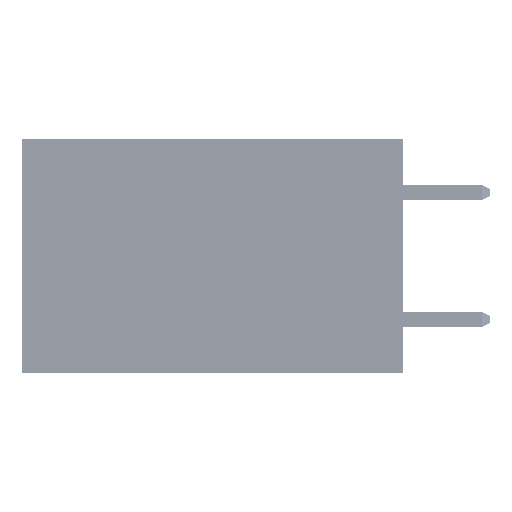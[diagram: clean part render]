
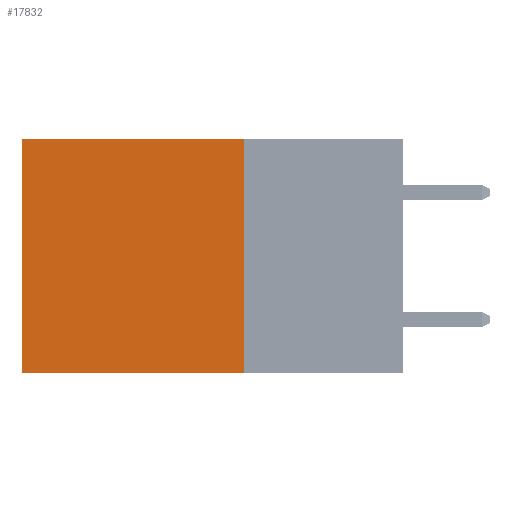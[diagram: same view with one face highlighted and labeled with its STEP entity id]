
A CAD part, left-side view. The second image highlights one B-rep face of the part: STEP entity #17832.
In plain terms, the highlighted planar face has unit normal (-1, 0, 0).
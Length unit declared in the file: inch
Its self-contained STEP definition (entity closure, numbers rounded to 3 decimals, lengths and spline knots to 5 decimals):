
#2434 = DIRECTION ( 'NONE',  ( 0., 1., 0. ) ) ;
#2795 = FACE_OUTER_BOUND ( 'NONE', #13570, .T. ) ;
#2867 = DIRECTION ( 'NONE',  ( 0., 0., -1. ) ) ;
#2980 = LINE ( 'NONE', #21636, #11363 ) ;
#3161 = ORIENTED_EDGE ( 'NONE', *, *, #35154, .F. ) ;
#4063 = ORIENTED_EDGE ( 'NONE', *, *, #6708, .T. ) ;
#6708 = EDGE_CURVE ( 'NONE', #41475, #39717, #28324, .T. ) ;
#8744 = CARTESIAN_POINT ( 'NONE',  ( 0.2875, 0.25, 0. ) ) ;
#10807 = VERTEX_POINT ( 'NONE', #38767 ) ;
#11097 = DIRECTION ( 'NONE',  ( 1., 0., 0. ) ) ;
#11363 = VECTOR ( 'NONE', #2434, 39.37008 ) ;
#11966 = DIRECTION ( 'NONE',  ( 0., 0., -1. ) ) ;
#13570 = EDGE_LOOP ( 'NONE', ( #26154, #39693, #3161, #4063 ) ) ;
#14655 = PLANE ( 'NONE',  #36126 ) ;
#15687 = VECTOR ( 'NONE', #39214, 39.37008 ) ;
#16543 = CARTESIAN_POINT ( 'NONE',  ( 0.2875, 0.25, 0. ) ) ;
#17832 = ADVANCED_FACE ( 'NONE', ( #2795 ), #14655, .F. ) ;
#20060 = VERTEX_POINT ( 'NONE', #35038 ) ;
#21636 = CARTESIAN_POINT ( 'NONE',  ( 0.2875, 0.25, -0.37 ) ) ;
#25729 = CARTESIAN_POINT ( 'NONE',  ( 0.2875, 0.6, 0. ) ) ;
#26066 = DIRECTION ( 'NONE',  ( 0., 0., -1. ) ) ;
#26154 = ORIENTED_EDGE ( 'NONE', *, *, #45832, .T. ) ;
#27317 = EDGE_CURVE ( 'NONE', #20060, #10807, #2980, .T. ) ;
#27403 = VECTOR ( 'NONE', #26066, 39.37008 ) ;
#28324 = LINE ( 'NONE', #8744, #15687 ) ;
#29808 = LINE ( 'NONE', #41364, #27403 ) ;
#30430 = LINE ( 'NONE', #35023, #31013 ) ;
#31013 = VECTOR ( 'NONE', #11966, 39.37008 ) ;
#35023 = CARTESIAN_POINT ( 'NONE',  ( 0.2875, 0.25, 0. ) ) ;
#35038 = CARTESIAN_POINT ( 'NONE',  ( 0.2875, 0.25, -0.37 ) ) ;
#35154 = EDGE_CURVE ( 'NONE', #41475, #20060, #30430, .T. ) ;
#36126 = AXIS2_PLACEMENT_3D ( 'NONE', #49220, #11097, #2867 ) ;
#38767 = CARTESIAN_POINT ( 'NONE',  ( 0.2875, 0.6, -0.37 ) ) ;
#39214 = DIRECTION ( 'NONE',  ( 0., 1., 0. ) ) ;
#39693 = ORIENTED_EDGE ( 'NONE', *, *, #27317, .F. ) ;
#39717 = VERTEX_POINT ( 'NONE', #25729 ) ;
#41364 = CARTESIAN_POINT ( 'NONE',  ( 0.2875, 0.6, 0. ) ) ;
#41475 = VERTEX_POINT ( 'NONE', #16543 ) ;
#45832 = EDGE_CURVE ( 'NONE', #39717, #10807, #29808, .T. ) ;
#49220 = CARTESIAN_POINT ( 'NONE',  ( 0.2875, 0.25, 0. ) ) ;
